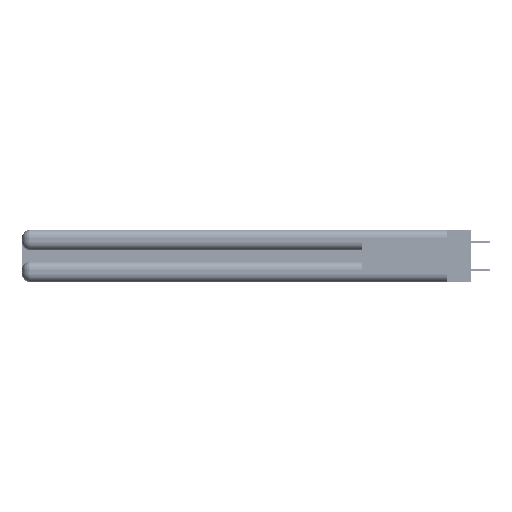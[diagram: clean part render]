
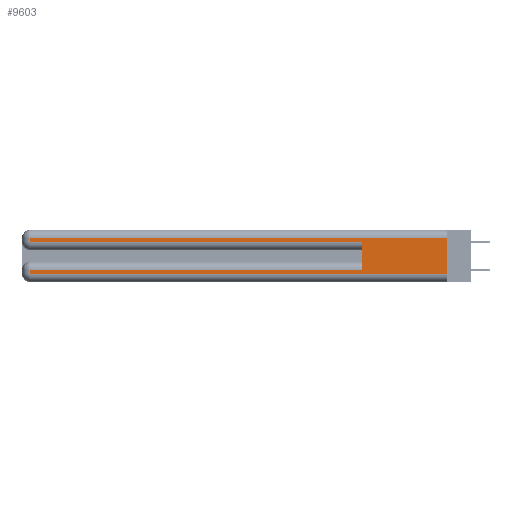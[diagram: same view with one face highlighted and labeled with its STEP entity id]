
A CAD part, left-side view. The second image highlights one B-rep face of the part: STEP entity #9603.
In plain terms, the highlighted planar face has unit normal (-1, 0, 0).
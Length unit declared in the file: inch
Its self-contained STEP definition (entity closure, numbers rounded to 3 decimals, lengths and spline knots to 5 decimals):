
#1301 = CARTESIAN_POINT ( 'NONE',  ( 0., 2.94, 0.085 ) ) ;
#1550 = ORIENTED_EDGE ( 'NONE', *, *, #11502, .T. ) ;
#1567 = DIRECTION ( 'NONE',  ( 0., 0., -1. ) ) ;
#1584 = LINE ( 'NONE', #11147, #9670 ) ;
#1651 = CARTESIAN_POINT ( 'NONE',  ( 0., 2.94, 0.37 ) ) ;
#2581 = LINE ( 'NONE', #16429, #34978 ) ;
#2633 = CARTESIAN_POINT ( 'NONE',  ( 0., 0., 0.37 ) ) ;
#2709 = VECTOR ( 'NONE', #28274, 39.37008 ) ;
#4004 = EDGE_CURVE ( 'NONE', #30708, #40588, #2581, .T. ) ;
#5937 = CARTESIAN_POINT ( 'NONE',  ( 0., 0., 0.37 ) ) ;
#6997 = DIRECTION ( 'NONE',  ( 1., 0., 0. ) ) ;
#9603 = ADVANCED_FACE ( 'NONE', ( #51310 ), #29248, .F. ) ;
#9670 = VECTOR ( 'NONE', #50545, 39.37008 ) ;
#9982 = LINE ( 'NONE', #5937, #43669 ) ;
#10347 = ORIENTED_EDGE ( 'NONE', *, *, #21980, .F. ) ;
#10743 = DIRECTION ( 'NONE',  ( 0., 0., -1. ) ) ;
#10990 = EDGE_CURVE ( 'NONE', #49908, #40517, #32751, .T. ) ;
#11147 = CARTESIAN_POINT ( 'NONE',  ( 0., 0.6, 0.145 ) ) ;
#11502 = EDGE_CURVE ( 'NONE', #41230, #30708, #51008, .T. ) ;
#13778 = ORIENTED_EDGE ( 'NONE', *, *, #39584, .F. ) ;
#16429 = CARTESIAN_POINT ( 'NONE',  ( 0., 0., 0.06 ) ) ;
#16832 = EDGE_CURVE ( 'NONE', #28687, #41230, #44242, .T. ) ;
#21980 = EDGE_CURVE ( 'NONE', #49908, #40588, #9982, .T. ) ;
#22088 = EDGE_LOOP ( 'NONE', ( #10347, #39069, #24014, #43903, #13778, #43881, #1550, #56719 ) ) ;
#23635 = LINE ( 'NONE', #1651, #2709 ) ;
#24014 = ORIENTED_EDGE ( 'NONE', *, *, #48522, .T. ) ;
#24920 = CARTESIAN_POINT ( 'NONE',  ( 0., 2.94, 0.285 ) ) ;
#25410 = DIRECTION ( 'NONE',  ( 0., -1., 0. ) ) ;
#25991 = EDGE_CURVE ( 'NONE', #37096, #36412, #56069, .T. ) ;
#26819 = DIRECTION ( 'NONE',  ( 0., 1., 0. ) ) ;
#27135 = AXIS2_PLACEMENT_3D ( 'NONE', #2633, #6997, #10743 ) ;
#28274 = DIRECTION ( 'NONE',  ( 0., 0., -1. ) ) ;
#28687 = VERTEX_POINT ( 'NONE', #32422 ) ;
#28828 = CARTESIAN_POINT ( 'NONE',  ( 0., 0.6, 0.285 ) ) ;
#28972 = DIRECTION ( 'NONE',  ( 0., 1., 0. ) ) ;
#29248 = PLANE ( 'NONE',  #27135 ) ;
#29803 = DIRECTION ( 'NONE',  ( 0., 0., -1. ) ) ;
#30708 = VERTEX_POINT ( 'NONE', #34108 ) ;
#32422 = CARTESIAN_POINT ( 'NONE',  ( 0., 0.6, 0.085 ) ) ;
#32751 = LINE ( 'NONE', #50440, #38382 ) ;
#34108 = CARTESIAN_POINT ( 'NONE',  ( 0., 2.94, 0.06 ) ) ;
#34978 = VECTOR ( 'NONE', #25410, 39.37008 ) ;
#36412 = VERTEX_POINT ( 'NONE', #28828 ) ;
#37096 = VERTEX_POINT ( 'NONE', #24920 ) ;
#38382 = VECTOR ( 'NONE', #28972, 39.37008 ) ;
#39069 = ORIENTED_EDGE ( 'NONE', *, *, #10990, .T. ) ;
#39584 = EDGE_CURVE ( 'NONE', #28687, #36412, #1584, .T. ) ;
#40517 = VERTEX_POINT ( 'NONE', #46683 ) ;
#40588 = VERTEX_POINT ( 'NONE', #46399 ) ;
#41230 = VERTEX_POINT ( 'NONE', #1301 ) ;
#43060 = VECTOR ( 'NONE', #29803, 39.37008 ) ;
#43669 = VECTOR ( 'NONE', #1567, 39.37008 ) ;
#43881 = ORIENTED_EDGE ( 'NONE', *, *, #16832, .T. ) ;
#43903 = ORIENTED_EDGE ( 'NONE', *, *, #25991, .T. ) ;
#44242 = LINE ( 'NONE', #49138, #51754 ) ;
#46399 = CARTESIAN_POINT ( 'NONE',  ( 0., 0., 0.06 ) ) ;
#46640 = CARTESIAN_POINT ( 'NONE',  ( 0., 2.94, 0.37 ) ) ;
#46683 = CARTESIAN_POINT ( 'NONE',  ( 0., 2.94, 0.31 ) ) ;
#48522 = EDGE_CURVE ( 'NONE', #40517, #37096, #23635, .T. ) ;
#49138 = CARTESIAN_POINT ( 'NONE',  ( 0., 0., 0.085 ) ) ;
#49908 = VERTEX_POINT ( 'NONE', #51776 ) ;
#50440 = CARTESIAN_POINT ( 'NONE',  ( 0., 0., 0.31 ) ) ;
#50481 = VECTOR ( 'NONE', #56356, 39.37008 ) ;
#50545 = DIRECTION ( 'NONE',  ( 0., 0., 1. ) ) ;
#51008 = LINE ( 'NONE', #46640, #43060 ) ;
#51310 = FACE_OUTER_BOUND ( 'NONE', #22088, .T. ) ;
#51754 = VECTOR ( 'NONE', #26819, 39.37008 ) ;
#51776 = CARTESIAN_POINT ( 'NONE',  ( 0., 0., 0.31 ) ) ;
#52012 = CARTESIAN_POINT ( 'NONE',  ( 0., 0., 0.285 ) ) ;
#56069 = LINE ( 'NONE', #52012, #50481 ) ;
#56356 = DIRECTION ( 'NONE',  ( 0., -1., 0. ) ) ;
#56719 = ORIENTED_EDGE ( 'NONE', *, *, #4004, .T. ) ;
